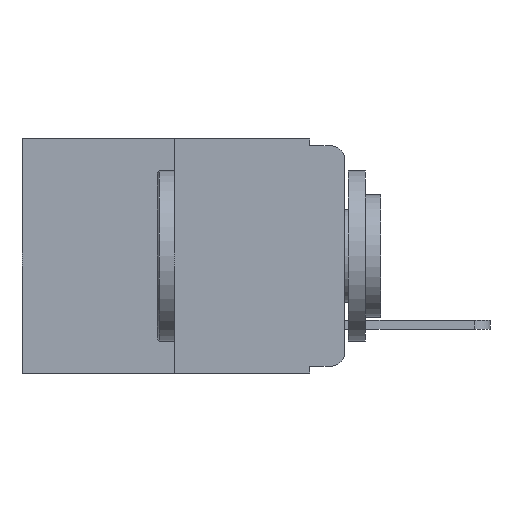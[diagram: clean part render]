
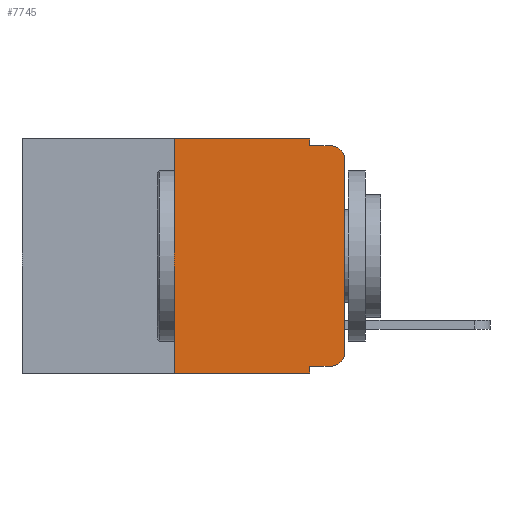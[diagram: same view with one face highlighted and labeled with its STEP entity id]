
A CAD part, left-side view. The second image highlights one B-rep face of the part: STEP entity #7745.
In plain terms, the highlighted planar face has unit normal (-1, 0, 0).
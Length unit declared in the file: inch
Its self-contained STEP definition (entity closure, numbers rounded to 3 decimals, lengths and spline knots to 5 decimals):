
#57 = VERTEX_POINT ( 'NONE', #10956 ) ;
#358 = VERTEX_POINT ( 'NONE', #6886 ) ;
#690 = ORIENTED_EDGE ( 'NONE', *, *, #3496, .F. ) ;
#1005 = CARTESIAN_POINT ( 'NONE',  ( 0., 0.051, 0. ) ) ;
#1119 = ORIENTED_EDGE ( 'NONE', *, *, #5556, .F. ) ;
#1190 = VERTEX_POINT ( 'NONE', #5711 ) ;
#1227 = LINE ( 'NONE', #12067, #6821 ) ;
#1531 = CIRCLE ( 'NONE', #13974, 0.02 ) ;
#2334 = DIRECTION ( 'NONE',  ( 0., 0., 1. ) ) ;
#2348 = CARTESIAN_POINT ( 'NONE',  ( 0., 0.02, -0.01 ) ) ;
#2704 = AXIS2_PLACEMENT_3D ( 'NONE', #11040, #12228, #14501 ) ;
#2756 = EDGE_CURVE ( 'NONE', #10752, #7792, #12082, .T. ) ;
#2842 = DIRECTION ( 'NONE',  ( 0., -1., 0. ) ) ;
#2992 = CARTESIAN_POINT ( 'NONE',  ( 0., 0.051, -0.333 ) ) ;
#2994 = VECTOR ( 'NONE', #6243, 39.37008 ) ;
#3379 = LINE ( 'NONE', #12212, #7696 ) ;
#3496 = EDGE_CURVE ( 'NONE', #4639, #358, #4417, .T. ) ;
#3585 = CARTESIAN_POINT ( 'NONE',  ( 0., 0.25, 0. ) ) ;
#3612 = LINE ( 'NONE', #7140, #12870 ) ;
#3831 = LINE ( 'NONE', #2992, #7252 ) ;
#3936 = ORIENTED_EDGE ( 'NONE', *, *, #13229, .T. ) ;
#3953 = VECTOR ( 'NONE', #13422, 39.37008 ) ;
#3988 = ORIENTED_EDGE ( 'NONE', *, *, #5298, .T. ) ;
#4267 = VECTOR ( 'NONE', #6611, 39.37008 ) ;
#4417 = LINE ( 'NONE', #4668, #8383 ) ;
#4639 = VERTEX_POINT ( 'NONE', #11991 ) ;
#4668 = CARTESIAN_POINT ( 'NONE',  ( 0., 0.051, 0. ) ) ;
#4672 = EDGE_CURVE ( 'NONE', #358, #12885, #14997, .T. ) ;
#5074 = DIRECTION ( 'NONE',  ( 0., 0., 1. ) ) ;
#5109 = CARTESIAN_POINT ( 'NONE',  ( 0., 0.051, -0.01 ) ) ;
#5298 = EDGE_CURVE ( 'NONE', #1190, #57, #3612, .T. ) ;
#5418 = DIRECTION ( 'NONE',  ( 0., 0., -1. ) ) ;
#5556 = EDGE_CURVE ( 'NONE', #9096, #6749, #1227, .T. ) ;
#5605 = EDGE_CURVE ( 'NONE', #9096, #7792, #13042, .T. ) ;
#5711 = CARTESIAN_POINT ( 'NONE',  ( 0., 0., -0.313 ) ) ;
#6215 = PLANE ( 'NONE',  #2704 ) ;
#6243 = DIRECTION ( 'NONE',  ( 0., -1., 0. ) ) ;
#6444 = CARTESIAN_POINT ( 'NONE',  ( 0., 0.02, -0.333 ) ) ;
#6611 = DIRECTION ( 'NONE',  ( 0., 0., -1. ) ) ;
#6625 = DIRECTION ( 'NONE',  ( -1., 0., 0. ) ) ;
#6749 = VERTEX_POINT ( 'NONE', #3585 ) ;
#6821 = VECTOR ( 'NONE', #5074, 39.37008 ) ;
#6886 = CARTESIAN_POINT ( 'NONE',  ( 0., 0.051, -0.01 ) ) ;
#7058 = ORIENTED_EDGE ( 'NONE', *, *, #8406, .F. ) ;
#7140 = CARTESIAN_POINT ( 'NONE',  ( 0., 0., 0. ) ) ;
#7252 = VECTOR ( 'NONE', #14761, 39.37008 ) ;
#7696 = VECTOR ( 'NONE', #2842, 39.37008 ) ;
#7739 = CARTESIAN_POINT ( 'NONE',  ( 0., 0.02, -0.03 ) ) ;
#7745 = ADVANCED_FACE ( 'NONE', ( #14817 ), #6215, .F. ) ;
#7792 = VERTEX_POINT ( 'NONE', #14545 ) ;
#8383 = VECTOR ( 'NONE', #14072, 39.37008 ) ;
#8406 = EDGE_CURVE ( 'NONE', #6749, #4639, #3379, .T. ) ;
#8432 = ORIENTED_EDGE ( 'NONE', *, *, #5605, .T. ) ;
#8884 = CARTESIAN_POINT ( 'NONE',  ( 0., 0.473, -0.343 ) ) ;
#9096 = VERTEX_POINT ( 'NONE', #9895 ) ;
#9895 = CARTESIAN_POINT ( 'NONE',  ( 0., 0.25, -0.343 ) ) ;
#9981 = EDGE_LOOP ( 'NONE', ( #3988, #3936, #11144, #690, #7058, #1119, #8432, #12316, #15008, #10997 ) ) ;
#9982 = CARTESIAN_POINT ( 'NONE',  ( 0., 0.02, -0.313 ) ) ;
#10565 = CARTESIAN_POINT ( 'NONE',  ( 0., 0.051, -0.333 ) ) ;
#10727 = CIRCLE ( 'NONE', #11436, 0.02 ) ;
#10752 = VERTEX_POINT ( 'NONE', #10565 ) ;
#10956 = CARTESIAN_POINT ( 'NONE',  ( 0., 0., -0.03 ) ) ;
#10997 = ORIENTED_EDGE ( 'NONE', *, *, #14426, .T. ) ;
#11040 = CARTESIAN_POINT ( 'NONE',  ( 0., 0.473, 0. ) ) ;
#11118 = DIRECTION ( 'NONE',  ( 0., 0., -1. ) ) ;
#11144 = ORIENTED_EDGE ( 'NONE', *, *, #4672, .F. ) ;
#11150 = DIRECTION ( 'NONE',  ( -1., 0., 0. ) ) ;
#11436 = AXIS2_PLACEMENT_3D ( 'NONE', #7739, #6625, #11118 ) ;
#11991 = CARTESIAN_POINT ( 'NONE',  ( 0., 0.051, 0. ) ) ;
#12067 = CARTESIAN_POINT ( 'NONE',  ( 0., 0.25, 0. ) ) ;
#12082 = LINE ( 'NONE', #1005, #4267 ) ;
#12212 = CARTESIAN_POINT ( 'NONE',  ( 0., 0.473, 0. ) ) ;
#12228 = DIRECTION ( 'NONE',  ( 1., 0., 0. ) ) ;
#12316 = ORIENTED_EDGE ( 'NONE', *, *, #2756, .F. ) ;
#12870 = VECTOR ( 'NONE', #2334, 39.37008 ) ;
#12885 = VERTEX_POINT ( 'NONE', #2348 ) ;
#13042 = LINE ( 'NONE', #8884, #3953 ) ;
#13211 = EDGE_CURVE ( 'NONE', #10752, #15033, #3831, .T. ) ;
#13229 = EDGE_CURVE ( 'NONE', #57, #12885, #10727, .T. ) ;
#13422 = DIRECTION ( 'NONE',  ( 0., -1., 0. ) ) ;
#13974 = AXIS2_PLACEMENT_3D ( 'NONE', #9982, #11150, #5418 ) ;
#14072 = DIRECTION ( 'NONE',  ( 0., 0., -1. ) ) ;
#14426 = EDGE_CURVE ( 'NONE', #15033, #1190, #1531, .T. ) ;
#14501 = DIRECTION ( 'NONE',  ( 0., 0., -1. ) ) ;
#14545 = CARTESIAN_POINT ( 'NONE',  ( 0., 0.051, -0.343 ) ) ;
#14761 = DIRECTION ( 'NONE',  ( 0., -1., 0. ) ) ;
#14817 = FACE_OUTER_BOUND ( 'NONE', #9981, .T. ) ;
#14997 = LINE ( 'NONE', #5109, #2994 ) ;
#15008 = ORIENTED_EDGE ( 'NONE', *, *, #13211, .T. ) ;
#15033 = VERTEX_POINT ( 'NONE', #6444 ) ;
